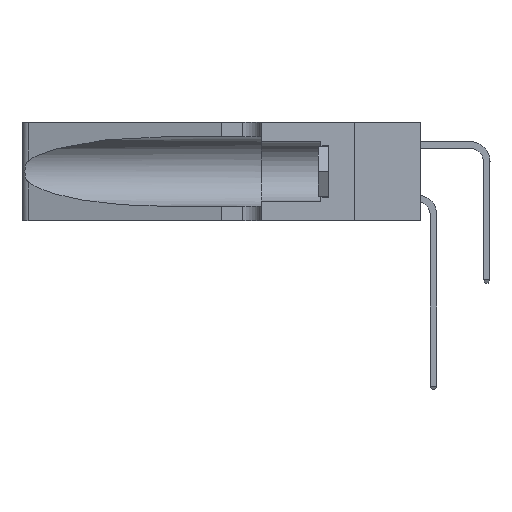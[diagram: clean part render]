
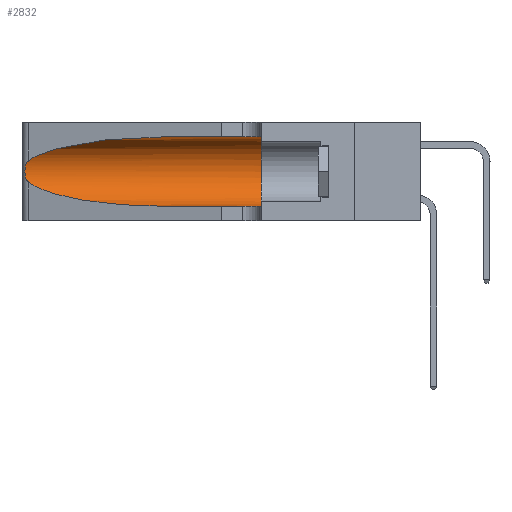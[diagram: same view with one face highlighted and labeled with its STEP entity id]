
A CAD part, left-side view. The second image highlights one B-rep face of the part: STEP entity #2832.
In plain terms, the highlighted cylindrical face has radius 3.308 mm (diameter 6.617 mm), a partial arc.
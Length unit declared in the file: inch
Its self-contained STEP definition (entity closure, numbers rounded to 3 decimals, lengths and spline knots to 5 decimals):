
#411 = CARTESIAN_POINT ( 'NONE',  ( 0.1305, 0.72297, 0.31525 ) ) ;
#437 =( BOUNDED_CURVE ( )  B_SPLINE_CURVE ( 3, ( #25998, #15948, #11969, #1681 ),
 .UNSPECIFIED., .F., .F. ) 
 B_SPLINE_CURVE_WITH_KNOTS ( ( 4, 4 ),
 ( 3.44316, 4.71239 ),
 .UNSPECIFIED. ) 
 CURVE ( )  GEOMETRIC_REPRESENTATION_ITEM ( )  RATIONAL_B_SPLINE_CURVE ( ( 1., 0.87, 0.87, 1. ) ) 
 REPRESENTATION_ITEM ( '' )  );
#791 =( BOUNDED_CURVE ( )  B_SPLINE_CURVE ( 3, ( #411, #8840, #4674, #12926 ),
 .UNSPECIFIED., .F., .F. ) 
 B_SPLINE_CURVE_WITH_KNOTS ( ( 4, 4 ),
 ( 1.5708, 2.84003 ),
 .UNSPECIFIED. ) 
 CURVE ( )  GEOMETRIC_REPRESENTATION_ITEM ( )  RATIONAL_B_SPLINE_CURVE ( ( 1., 0.87, 0.87, 1. ) ) 
 REPRESENTATION_ITEM ( '' )  );
#1367 = VECTOR ( 'NONE', #4039, 39.37008 ) ;
#1512 = CARTESIAN_POINT ( 'NONE',  ( 0.26075, 1.23896, 0.178 ) ) ;
#1552 = LINE ( 'NONE', #23986, #11896 ) ;
#1681 = CARTESIAN_POINT ( 'NONE',  ( 0.1305, 0.72297, 0.05475 ) ) ;
#2000 = VERTEX_POINT ( 'NONE', #11386 ) ;
#2832 = ADVANCED_FACE ( 'NONE', ( #11251 ), #10006, .F. ) ;
#3441 = CARTESIAN_POINT ( 'NONE',  ( 0.1305, 0.35, 0.31525 ) ) ;
#3564 = CARTESIAN_POINT ( 'NONE',  ( 0.25487, 1.22718, 0.22369 ) ) ;
#3653 = CARTESIAN_POINT ( 'NONE',  ( 0.25856, 1.23593, 0.16098 ) ) ;
#3888 = EDGE_CURVE ( 'NONE', #7718, #14070, #791, .T. ) ;
#4039 = DIRECTION ( 'NONE',  ( 0., -1., 0. ) ) ;
#4674 = CARTESIAN_POINT ( 'NONE',  ( 0.2373, 1.15595, 0.28018 ) ) ;
#4932 = EDGE_CURVE ( 'NONE', #19864, #20288, #437, .T. ) ;
#5605 = DIRECTION ( 'NONE',  ( 0., 1., 0. ) ) ;
#5709 = CARTESIAN_POINT ( 'NONE',  ( 0.25639, 1.23186, 0.15144 ) ) ;
#5993 = EDGE_CURVE ( 'NONE', #20288, #2000, #6916, .T. ) ;
#6302 = B_SPLINE_CURVE_WITH_KNOTS ( 'NONE', 3,
 ( #3564, #17795, #9823, #23858, #11811, #25855, #13906, #1512, #15888, #3653, #17880, #5709, #19921, #7798 ),
 .UNSPECIFIED., .F., .F.,
 ( 4, 2, 2, 2, 2, 2, 4 ),
 ( 0., 0.00027, 0.00053, 0.00107, 0.0016, 0.00187, 0.00214 ),
 .UNSPECIFIED. ) ;
#6916 = LINE ( 'NONE', #16259, #1367 ) ;
#6930 = ORIENTED_EDGE ( 'NONE', *, *, #3888, .T. ) ;
#7155 = VERTEX_POINT ( 'NONE', #3441 ) ;
#7229 = CARTESIAN_POINT ( 'NONE',  ( 0.1305, 1.61858, 0.185 ) ) ;
#7247 = ORIENTED_EDGE ( 'NONE', *, *, #23128, .T. ) ;
#7283 = ORIENTED_EDGE ( 'NONE', *, *, #4932, .T. ) ;
#7351 = ORIENTED_EDGE ( 'NONE', *, *, #5993, .T. ) ;
#7718 = VERTEX_POINT ( 'NONE', #25808 ) ;
#7779 = ORIENTED_EDGE ( 'NONE', *, *, #14639, .F. ) ;
#7798 = CARTESIAN_POINT ( 'NONE',  ( 0.25487, 1.22718, 0.14631 ) ) ;
#7945 = AXIS2_PLACEMENT_3D ( 'NONE', #17772, #5605, #19815 ) ;
#8840 = CARTESIAN_POINT ( 'NONE',  ( 0.18966, 0.96281, 0.31525 ) ) ;
#9823 = CARTESIAN_POINT ( 'NONE',  ( 0.25639, 1.23184, 0.21858 ) ) ;
#10006 = CYLINDRICAL_SURFACE ( 'NONE', #18440, 0.13025 ) ;
#10344 = CARTESIAN_POINT ( 'NONE',  ( 0.25487, 1.22718, 0.22369 ) ) ;
#11251 = FACE_OUTER_BOUND ( 'NONE', #17547, .T. ) ;
#11386 = CARTESIAN_POINT ( 'NONE',  ( 0.1305, 0.35, 0.05475 ) ) ;
#11811 = CARTESIAN_POINT ( 'NONE',  ( 0.25854, 1.2359, 0.20912 ) ) ;
#11896 = VECTOR ( 'NONE', #25985, 39.37008 ) ;
#11932 = ORIENTED_EDGE ( 'NONE', *, *, #23776, .F. ) ;
#11969 = CARTESIAN_POINT ( 'NONE',  ( 0.18966, 0.96281, 0.05475 ) ) ;
#12926 = CARTESIAN_POINT ( 'NONE',  ( 0.25487, 1.22718, 0.22369 ) ) ;
#13906 = CARTESIAN_POINT ( 'NONE',  ( 0.26075, 1.23896, 0.19203 ) ) ;
#14070 = VERTEX_POINT ( 'NONE', #10344 ) ;
#14639 = EDGE_CURVE ( 'NONE', #7155, #2000, #19652, .T. ) ;
#15888 = CARTESIAN_POINT ( 'NONE',  ( 0.26017, 1.23833, 0.17102 ) ) ;
#15948 = CARTESIAN_POINT ( 'NONE',  ( 0.2373, 1.15595, 0.08982 ) ) ;
#15986 = CARTESIAN_POINT ( 'NONE',  ( 0.25487, 1.22718, 0.14631 ) ) ;
#16259 = CARTESIAN_POINT ( 'NONE',  ( 0.1305, 1.61858, 0.05475 ) ) ;
#17352 = DIRECTION ( 'NONE',  ( 0., 0., -1. ) ) ;
#17547 = EDGE_LOOP ( 'NONE', ( #6930, #7247, #7283, #7351, #7779, #11932 ) ) ;
#17772 = CARTESIAN_POINT ( 'NONE',  ( 0.1305, 0.35, 0.185 ) ) ;
#17795 = CARTESIAN_POINT ( 'NONE',  ( 0.25555, 1.22994, 0.2215 ) ) ;
#17880 = CARTESIAN_POINT ( 'NONE',  ( 0.25789, 1.23486, 0.15765 ) ) ;
#18440 = AXIS2_PLACEMENT_3D ( 'NONE', #7229, #23409, #17352 ) ;
#19652 = CIRCLE ( 'NONE', #7945, 0.13025 ) ;
#19815 = DIRECTION ( 'NONE',  ( 0., 0., 1. ) ) ;
#19864 = VERTEX_POINT ( 'NONE', #15986 ) ;
#19921 = CARTESIAN_POINT ( 'NONE',  ( 0.25555, 1.22993, 0.14849 ) ) ;
#20288 = VERTEX_POINT ( 'NONE', #25324 ) ;
#23128 = EDGE_CURVE ( 'NONE', #14070, #19864, #6302, .T. ) ;
#23409 = DIRECTION ( 'NONE',  ( 0., -1., 0. ) ) ;
#23776 = EDGE_CURVE ( 'NONE', #7718, #7155, #1552, .T. ) ;
#23858 = CARTESIAN_POINT ( 'NONE',  ( 0.25787, 1.23484, 0.2124 ) ) ;
#23986 = CARTESIAN_POINT ( 'NONE',  ( 0.1305, 1.61858, 0.31525 ) ) ;
#25324 = CARTESIAN_POINT ( 'NONE',  ( 0.1305, 0.72297, 0.05475 ) ) ;
#25808 = CARTESIAN_POINT ( 'NONE',  ( 0.1305, 0.72297, 0.31525 ) ) ;
#25855 = CARTESIAN_POINT ( 'NONE',  ( 0.26018, 1.23835, 0.19895 ) ) ;
#25985 = DIRECTION ( 'NONE',  ( 0., -1., 0. ) ) ;
#25998 = CARTESIAN_POINT ( 'NONE',  ( 0.25487, 1.22718, 0.14631 ) ) ;
